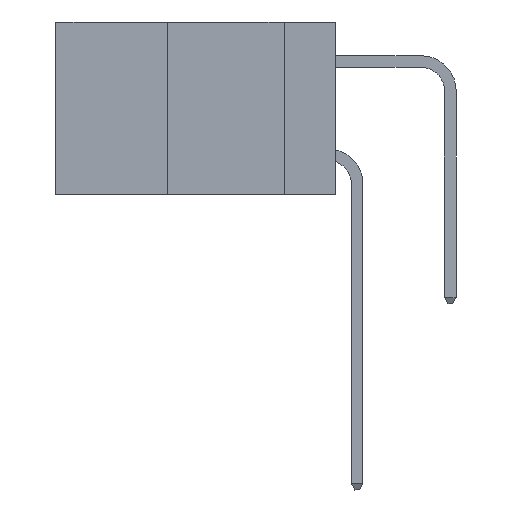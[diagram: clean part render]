
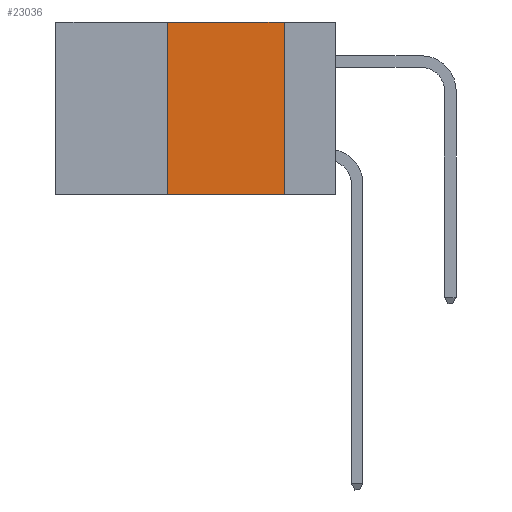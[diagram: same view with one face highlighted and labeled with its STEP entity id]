
A CAD part, left-side view. The second image highlights one B-rep face of the part: STEP entity #23036.
In plain terms, the highlighted planar face has unit normal (-1, 0, 0).
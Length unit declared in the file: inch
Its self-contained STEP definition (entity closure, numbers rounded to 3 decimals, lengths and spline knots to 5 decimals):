
#571 = CARTESIAN_POINT ( 'NONE',  ( 0., 0.11, -0.37 ) ) ;
#751 = EDGE_CURVE ( 'NONE', #2970, #20972, #14806, .T. ) ;
#1267 = EDGE_CURVE ( 'NONE', #3230, #20972, #14998, .T. ) ;
#2568 = ORIENTED_EDGE ( 'NONE', *, *, #14703, .F. ) ;
#2648 = CARTESIAN_POINT ( 'NONE',  ( 0., 0.6, -0.37 ) ) ;
#2970 = VERTEX_POINT ( 'NONE', #7673 ) ;
#3230 = VERTEX_POINT ( 'NONE', #22391 ) ;
#7673 = CARTESIAN_POINT ( 'NONE',  ( 0., 0.11, 0. ) ) ;
#8845 = VECTOR ( 'NONE', #26042, 39.37008 ) ;
#9379 = VECTOR ( 'NONE', #15041, 39.37008 ) ;
#9679 = CARTESIAN_POINT ( 'NONE',  ( 0., 0.36, 0. ) ) ;
#9912 = LINE ( 'NONE', #12758, #23876 ) ;
#11074 = PLANE ( 'NONE',  #12859 ) ;
#12758 = CARTESIAN_POINT ( 'NONE',  ( 0., 0.6, 0. ) ) ;
#12859 = AXIS2_PLACEMENT_3D ( 'NONE', #17611, #22406, #27028 ) ;
#13813 = ORIENTED_EDGE ( 'NONE', *, *, #18184, .F. ) ;
#14703 = EDGE_CURVE ( 'NONE', #3230, #17099, #19814, .T. ) ;
#14806 = LINE ( 'NONE', #17329, #9379 ) ;
#14998 = LINE ( 'NONE', #2648, #8845 ) ;
#15041 = DIRECTION ( 'NONE',  ( 0., 0., -1. ) ) ;
#15102 = DIRECTION ( 'NONE',  ( 0., -1., 0. ) ) ;
#17099 = VERTEX_POINT ( 'NONE', #28093 ) ;
#17329 = CARTESIAN_POINT ( 'NONE',  ( 0., 0.11, 0. ) ) ;
#17611 = CARTESIAN_POINT ( 'NONE',  ( 0., 0.6, 0. ) ) ;
#18184 = EDGE_CURVE ( 'NONE', #17099, #2970, #9912, .T. ) ;
#19814 = LINE ( 'NONE', #9679, #20547 ) ;
#20547 = VECTOR ( 'NONE', #25562, 39.37008 ) ;
#20972 = VERTEX_POINT ( 'NONE', #571 ) ;
#22391 = CARTESIAN_POINT ( 'NONE',  ( 0., 0.36, -0.37 ) ) ;
#22406 = DIRECTION ( 'NONE',  ( 1., 0., 0. ) ) ;
#22953 = EDGE_LOOP ( 'NONE', ( #23335, #13813, #2568, #23882 ) ) ;
#23036 = ADVANCED_FACE ( 'NONE', ( #26662 ), #11074, .F. ) ;
#23335 = ORIENTED_EDGE ( 'NONE', *, *, #751, .F. ) ;
#23876 = VECTOR ( 'NONE', #15102, 39.37008 ) ;
#23882 = ORIENTED_EDGE ( 'NONE', *, *, #1267, .T. ) ;
#25562 = DIRECTION ( 'NONE',  ( 0., 0., 1. ) ) ;
#26042 = DIRECTION ( 'NONE',  ( 0., -1., 0. ) ) ;
#26662 = FACE_OUTER_BOUND ( 'NONE', #22953, .T. ) ;
#27028 = DIRECTION ( 'NONE',  ( 0., 0., -1. ) ) ;
#28093 = CARTESIAN_POINT ( 'NONE',  ( 0., 0.36, 0. ) ) ;
